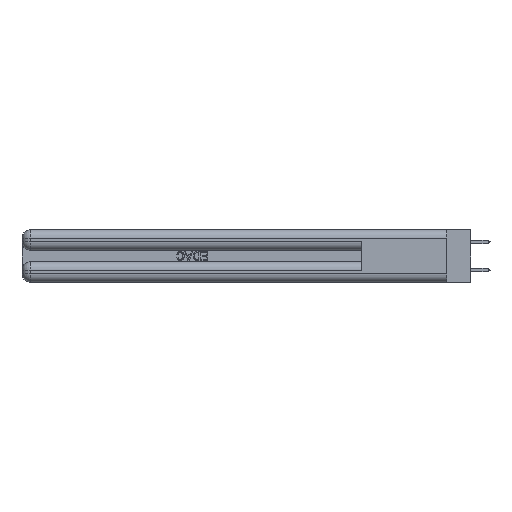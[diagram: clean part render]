
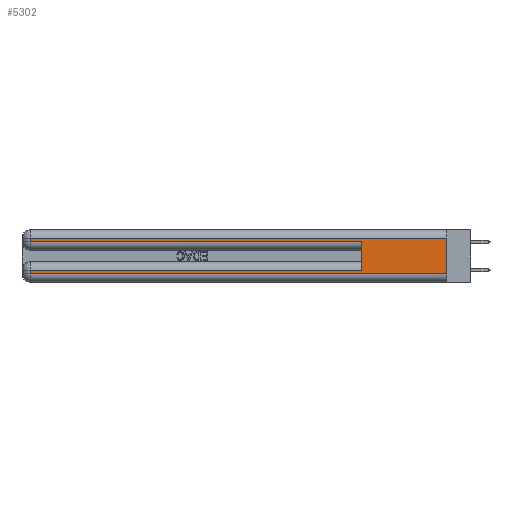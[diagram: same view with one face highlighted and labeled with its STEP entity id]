
A CAD part, left-side view. The second image highlights one B-rep face of the part: STEP entity #5302.
In plain terms, the highlighted planar face has unit normal (-1, 0, 0).
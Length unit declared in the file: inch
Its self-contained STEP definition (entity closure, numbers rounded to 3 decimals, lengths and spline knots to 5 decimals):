
#92 = EDGE_CURVE ( 'NONE', #201, #41890, #2507, .T. ) ;
#149 = VECTOR ( 'NONE', #17089, 39.37008 ) ;
#201 = VERTEX_POINT ( 'NONE', #40094 ) ;
#432 = ORIENTED_EDGE ( 'NONE', *, *, #38059, .T. ) ;
#1402 = CARTESIAN_POINT ( 'NONE',  ( 0., 0., 0.31 ) ) ;
#2448 = CARTESIAN_POINT ( 'NONE',  ( 0., 0., 0.37 ) ) ;
#2507 = LINE ( 'NONE', #13323, #149 ) ;
#2935 = CARTESIAN_POINT ( 'NONE',  ( 0., 2.94, 0.37 ) ) ;
#3893 = EDGE_CURVE ( 'NONE', #25163, #18600, #7597, .T. ) ;
#4251 = EDGE_CURVE ( 'NONE', #27754, #41890, #33134, .T. ) ;
#5159 = DIRECTION ( 'NONE',  ( 0., 1., 0. ) ) ;
#5167 = FACE_OUTER_BOUND ( 'NONE', #11282, .T. ) ;
#5302 = ADVANCED_FACE ( 'NONE', ( #5167 ), #33977, .F. ) ;
#5992 = CARTESIAN_POINT ( 'NONE',  ( 0., 0.6, 0.285 ) ) ;
#6018 = CARTESIAN_POINT ( 'NONE',  ( 0., 2.94, 0.085 ) ) ;
#7597 = LINE ( 'NONE', #37516, #9938 ) ;
#9121 = ORIENTED_EDGE ( 'NONE', *, *, #3893, .T. ) ;
#9938 = VECTOR ( 'NONE', #41238, 39.37008 ) ;
#10855 = ORIENTED_EDGE ( 'NONE', *, *, #38422, .T. ) ;
#10974 = CARTESIAN_POINT ( 'NONE',  ( 0., 2.94, 0.31 ) ) ;
#11282 = EDGE_LOOP ( 'NONE', ( #39315, #10855, #34105, #9121, #28910, #432, #13808, #33547 ) ) ;
#11446 = CARTESIAN_POINT ( 'NONE',  ( 0., 0., 0.31 ) ) ;
#11611 = EDGE_CURVE ( 'NONE', #37537, #201, #44256, .T. ) ;
#13323 = CARTESIAN_POINT ( 'NONE',  ( 0., 0., 0.06 ) ) ;
#13626 = VECTOR ( 'NONE', #5159, 39.37008 ) ;
#13808 = ORIENTED_EDGE ( 'NONE', *, *, #11611, .T. ) ;
#16049 = CARTESIAN_POINT ( 'NONE',  ( 0., 0., 0.085 ) ) ;
#16993 = CARTESIAN_POINT ( 'NONE',  ( 0., 2.94, 0.37 ) ) ;
#17089 = DIRECTION ( 'NONE',  ( 0., -1., 0. ) ) ;
#17484 = VECTOR ( 'NONE', #42925, 39.37008 ) ;
#18600 = VERTEX_POINT ( 'NONE', #5992 ) ;
#19231 = DIRECTION ( 'NONE',  ( 1., 0., 0. ) ) ;
#20302 = CARTESIAN_POINT ( 'NONE',  ( 0., 0.6, 0.145 ) ) ;
#20484 = CARTESIAN_POINT ( 'NONE',  ( 0., 2.94, 0.285 ) ) ;
#21940 = EDGE_CURVE ( 'NONE', #23454, #25163, #45877, .T. ) ;
#22106 = VECTOR ( 'NONE', #35839, 39.37008 ) ;
#23454 = VERTEX_POINT ( 'NONE', #10974 ) ;
#23929 = LINE ( 'NONE', #20302, #43664 ) ;
#24676 = LINE ( 'NONE', #16049, #13626 ) ;
#25163 = VERTEX_POINT ( 'NONE', #20484 ) ;
#26990 = VERTEX_POINT ( 'NONE', #33767 ) ;
#27754 = VERTEX_POINT ( 'NONE', #1402 ) ;
#27761 = CARTESIAN_POINT ( 'NONE',  ( 0., 0., 0.06 ) ) ;
#28910 = ORIENTED_EDGE ( 'NONE', *, *, #32179, .F. ) ;
#29287 = LINE ( 'NONE', #11446, #46659 ) ;
#30123 = DIRECTION ( 'NONE',  ( 0., 1., 0. ) ) ;
#32179 = EDGE_CURVE ( 'NONE', #26990, #18600, #23929, .T. ) ;
#32612 = DIRECTION ( 'NONE',  ( 0., 0., -1. ) ) ;
#33134 = LINE ( 'NONE', #2448, #22106 ) ;
#33547 = ORIENTED_EDGE ( 'NONE', *, *, #92, .T. ) ;
#33767 = CARTESIAN_POINT ( 'NONE',  ( 0., 0.6, 0.085 ) ) ;
#33977 = PLANE ( 'NONE',  #41012 ) ;
#34105 = ORIENTED_EDGE ( 'NONE', *, *, #21940, .T. ) ;
#35839 = DIRECTION ( 'NONE',  ( 0., 0., -1. ) ) ;
#37516 = CARTESIAN_POINT ( 'NONE',  ( 0., 0., 0.285 ) ) ;
#37537 = VERTEX_POINT ( 'NONE', #6018 ) ;
#38059 = EDGE_CURVE ( 'NONE', #26990, #37537, #24676, .T. ) ;
#38422 = EDGE_CURVE ( 'NONE', #27754, #23454, #29287, .T. ) ;
#39315 = ORIENTED_EDGE ( 'NONE', *, *, #4251, .F. ) ;
#40094 = CARTESIAN_POINT ( 'NONE',  ( 0., 2.94, 0.06 ) ) ;
#41012 = AXIS2_PLACEMENT_3D ( 'NONE', #41448, #19231, #45139 ) ;
#41238 = DIRECTION ( 'NONE',  ( 0., -1., 0. ) ) ;
#41448 = CARTESIAN_POINT ( 'NONE',  ( 0., 0., 0.37 ) ) ;
#41890 = VERTEX_POINT ( 'NONE', #27761 ) ;
#42925 = DIRECTION ( 'NONE',  ( 0., 0., -1. ) ) ;
#43116 = VECTOR ( 'NONE', #32612, 39.37008 ) ;
#43664 = VECTOR ( 'NONE', #46223, 39.37008 ) ;
#44256 = LINE ( 'NONE', #2935, #43116 ) ;
#45139 = DIRECTION ( 'NONE',  ( 0., 0., -1. ) ) ;
#45877 = LINE ( 'NONE', #16993, #17484 ) ;
#46223 = DIRECTION ( 'NONE',  ( 0., 0., 1. ) ) ;
#46659 = VECTOR ( 'NONE', #30123, 39.37008 ) ;
